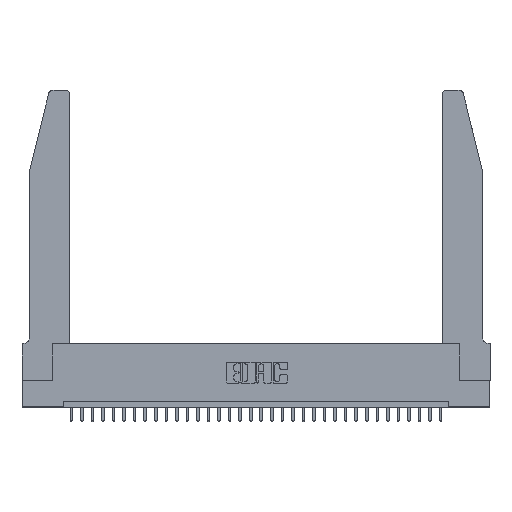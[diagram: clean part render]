
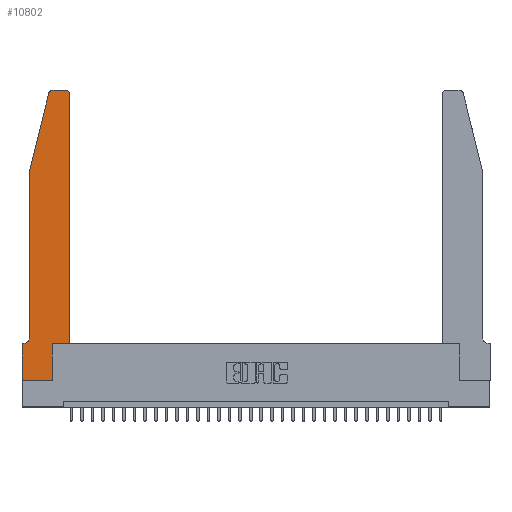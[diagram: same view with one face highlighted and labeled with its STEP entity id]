
A CAD part, top view. The second image highlights one B-rep face of the part: STEP entity #10802.
In plain terms, the highlighted planar face has unit normal (0, 0, 1).
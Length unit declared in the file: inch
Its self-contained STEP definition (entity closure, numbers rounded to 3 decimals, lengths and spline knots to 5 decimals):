
#451 = FACE_OUTER_BOUND ( 'NONE', #29795, .T. ) ;
#665 = DIRECTION ( 'NONE',  ( 1., 0., 0. ) ) ;
#1208 = CARTESIAN_POINT ( 'NONE',  ( 0., 0., 0.37 ) ) ;
#1330 = VECTOR ( 'NONE', #31803, 39.37008 ) ;
#1458 = LINE ( 'NONE', #11504, #6592 ) ;
#1498 = EDGE_CURVE ( 'NONE', #8237, #25740, #8897, .T. ) ;
#1564 = CARTESIAN_POINT ( 'NONE',  ( 0.284, 2.72, 0.37 ) ) ;
#2473 = CARTESIAN_POINT ( 'NONE',  ( 0.2865, 0.35, 0.37 ) ) ;
#2876 = CARTESIAN_POINT ( 'NONE',  ( 0.4205, 2.75, 0.37 ) ) ;
#3029 = EDGE_CURVE ( 'NONE', #7109, #3863, #8797, .T. ) ;
#3073 = DIRECTION ( 'NONE',  ( 0., 0., 1. ) ) ;
#3203 = ORIENTED_EDGE ( 'NONE', *, *, #6358, .T. ) ;
#3632 = VECTOR ( 'NONE', #28051, 39.37008 ) ;
#3680 = EDGE_CURVE ( 'NONE', #12572, #7109, #15431, .T. ) ;
#3863 = VERTEX_POINT ( 'NONE', #2876 ) ;
#4445 = EDGE_CURVE ( 'NONE', #31899, #6342, #7865, .T. ) ;
#4623 = ORIENTED_EDGE ( 'NONE', *, *, #17757, .T. ) ;
#4639 = CARTESIAN_POINT ( 'NONE',  ( 0., 0., 0.37 ) ) ;
#5133 = VECTOR ( 'NONE', #20502, 39.37008 ) ;
#5402 = CARTESIAN_POINT ( 'NONE',  ( 0.0755, 2., 0.37 ) ) ;
#5585 = LINE ( 'NONE', #27454, #13978 ) ;
#5734 = ORIENTED_EDGE ( 'NONE', *, *, #11113, .T. ) ;
#6342 = VERTEX_POINT ( 'NONE', #15612 ) ;
#6358 = EDGE_CURVE ( 'NONE', #27965, #6987, #21297, .T. ) ;
#6390 = ORIENTED_EDGE ( 'NONE', *, *, #1498, .T. ) ;
#6541 = DIRECTION ( 'NONE',  ( 1., 0., 0. ) ) ;
#6592 = VECTOR ( 'NONE', #13815, 39.37008 ) ;
#6987 = VERTEX_POINT ( 'NONE', #24351 ) ;
#7109 = VERTEX_POINT ( 'NONE', #26848 ) ;
#7865 = LINE ( 'NONE', #26469, #22881 ) ;
#8096 = VECTOR ( 'NONE', #15137, 39.37008 ) ;
#8237 = VERTEX_POINT ( 'NONE', #1208 ) ;
#8797 = CIRCLE ( 'NONE', #13568, 0.03 ) ;
#8897 = LINE ( 'NONE', #4639, #31772 ) ;
#8945 = EDGE_CURVE ( 'NONE', #24243, #10472, #30997, .T. ) ;
#9319 = DIRECTION ( 'NONE',  ( 0., 0., 1. ) ) ;
#9428 = DIRECTION ( 'NONE',  ( 1., 0., 0. ) ) ;
#10472 = VERTEX_POINT ( 'NONE', #11998 ) ;
#10667 = ORIENTED_EDGE ( 'NONE', *, *, #4445, .T. ) ;
#10802 = ADVANCED_FACE ( 'NONE', ( #451 ), #31542, .T. ) ;
#10900 = ORIENTED_EDGE ( 'NONE', *, *, #27400, .T. ) ;
#11113 = EDGE_CURVE ( 'NONE', #25740, #26515, #5585, .T. ) ;
#11221 = DIRECTION ( 'NONE',  ( 1., 0., 0. ) ) ;
#11504 = CARTESIAN_POINT ( 'NONE',  ( 0.0755, 2., 0.37 ) ) ;
#11998 = CARTESIAN_POINT ( 'NONE',  ( 0.0755, 0.42, 0.37 ) ) ;
#12572 = VERTEX_POINT ( 'NONE', #23855 ) ;
#13005 = CARTESIAN_POINT ( 'NONE',  ( 0.0055, 0.35, 0.37 ) ) ;
#13304 = ORIENTED_EDGE ( 'NONE', *, *, #8945, .T. ) ;
#13366 = VECTOR ( 'NONE', #6541, 39.37008 ) ;
#13568 = AXIS2_PLACEMENT_3D ( 'NONE', #28246, #3073, #665 ) ;
#13815 = DIRECTION ( 'NONE',  ( -0.239, -0.971, 0. ) ) ;
#13978 = VECTOR ( 'NONE', #30307, 39.37008 ) ;
#14035 = CARTESIAN_POINT ( 'NONE',  ( 0.284, 2.75, 0.37 ) ) ;
#14334 = CIRCLE ( 'NONE', #30032, 0.07 ) ;
#15137 = DIRECTION ( 'NONE',  ( 0., -1., 0. ) ) ;
#15431 = LINE ( 'NONE', #23204, #5133 ) ;
#15490 = ORIENTED_EDGE ( 'NONE', *, *, #19650, .T. ) ;
#15612 = CARTESIAN_POINT ( 'NONE',  ( 0., 0.35, 0.37 ) ) ;
#16112 = CARTESIAN_POINT ( 'NONE',  ( 0.0055, 0.42, 0.37 ) ) ;
#16457 = AXIS2_PLACEMENT_3D ( 'NONE', #32282, #28733, #11221 ) ;
#17757 = EDGE_CURVE ( 'NONE', #10472, #31899, #14334, .T. ) ;
#19650 = EDGE_CURVE ( 'NONE', #6987, #24243, #1458, .T. ) ;
#20502 = DIRECTION ( 'NONE',  ( 0., 1., 0. ) ) ;
#21024 = DIRECTION ( 'NONE',  ( 0., 0., -1. ) ) ;
#21297 = CIRCLE ( 'NONE', #32598, 0.03 ) ;
#21918 = EDGE_CURVE ( 'NONE', #6342, #8237, #32090, .T. ) ;
#22000 = LINE ( 'NONE', #29375, #13366 ) ;
#22292 = CARTESIAN_POINT ( 'NONE',  ( 0.2865, 0., 0.37 ) ) ;
#22881 = VECTOR ( 'NONE', #24040, 39.37008 ) ;
#22966 = ORIENTED_EDGE ( 'NONE', *, *, #3029, .T. ) ;
#23204 = CARTESIAN_POINT ( 'NONE',  ( 0.4505, 0.35, 0.37 ) ) ;
#23855 = CARTESIAN_POINT ( 'NONE',  ( 0.4505, 0.35, 0.37 ) ) ;
#24040 = DIRECTION ( 'NONE',  ( -1., 0., 0. ) ) ;
#24243 = VERTEX_POINT ( 'NONE', #27750 ) ;
#24351 = CARTESIAN_POINT ( 'NONE',  ( 0.25487, 2.72718, 0.37 ) ) ;
#24922 = ORIENTED_EDGE ( 'NONE', *, *, #29316, .T. ) ;
#25499 = ORIENTED_EDGE ( 'NONE', *, *, #3680, .T. ) ;
#25740 = VERTEX_POINT ( 'NONE', #22292 ) ;
#26469 = CARTESIAN_POINT ( 'NONE',  ( 0.0755, 0.35, 0.37 ) ) ;
#26515 = VERTEX_POINT ( 'NONE', #2473 ) ;
#26642 = LINE ( 'NONE', #32004, #1330 ) ;
#26848 = CARTESIAN_POINT ( 'NONE',  ( 0.4505, 2.72, 0.37 ) ) ;
#27020 = DIRECTION ( 'NONE',  ( -1., 0., 0. ) ) ;
#27400 = EDGE_CURVE ( 'NONE', #26515, #12572, #22000, .T. ) ;
#27420 = CARTESIAN_POINT ( 'NONE',  ( 0., 0., 0.37 ) ) ;
#27454 = CARTESIAN_POINT ( 'NONE',  ( 0.2865, 0.35, 0.37 ) ) ;
#27639 = ORIENTED_EDGE ( 'NONE', *, *, #21918, .T. ) ;
#27750 = CARTESIAN_POINT ( 'NONE',  ( 0.0755, 2., 0.37 ) ) ;
#27965 = VERTEX_POINT ( 'NONE', #14035 ) ;
#28051 = DIRECTION ( 'NONE',  ( 0., -1., 0. ) ) ;
#28246 = CARTESIAN_POINT ( 'NONE',  ( 0.4205, 2.72, 0.37 ) ) ;
#28733 = DIRECTION ( 'NONE',  ( 0., 0., 1. ) ) ;
#29316 = EDGE_CURVE ( 'NONE', #3863, #27965, #26642, .T. ) ;
#29375 = CARTESIAN_POINT ( 'NONE',  ( 0.4505, 0.35, 0.37 ) ) ;
#29795 = EDGE_LOOP ( 'NONE', ( #24922, #3203, #15490, #13304, #4623, #10667, #27639, #6390, #5734, #10900, #25499, #22966 ) ) ;
#30032 = AXIS2_PLACEMENT_3D ( 'NONE', #16112, #21024, #27020 ) ;
#30307 = DIRECTION ( 'NONE',  ( 0., 1., 0. ) ) ;
#30997 = LINE ( 'NONE', #5402, #8096 ) ;
#31542 = PLANE ( 'NONE',  #16457 ) ;
#31772 = VECTOR ( 'NONE', #32457, 39.37008 ) ;
#31803 = DIRECTION ( 'NONE',  ( -1., 0., 0. ) ) ;
#31899 = VERTEX_POINT ( 'NONE', #13005 ) ;
#32004 = CARTESIAN_POINT ( 'NONE',  ( 0.2605, 2.75, 0.37 ) ) ;
#32090 = LINE ( 'NONE', #27420, #3632 ) ;
#32282 = CARTESIAN_POINT ( 'NONE',  ( 0., 0.35, 0.37 ) ) ;
#32457 = DIRECTION ( 'NONE',  ( 1., 0., 0. ) ) ;
#32598 = AXIS2_PLACEMENT_3D ( 'NONE', #1564, #9319, #9428 ) ;
